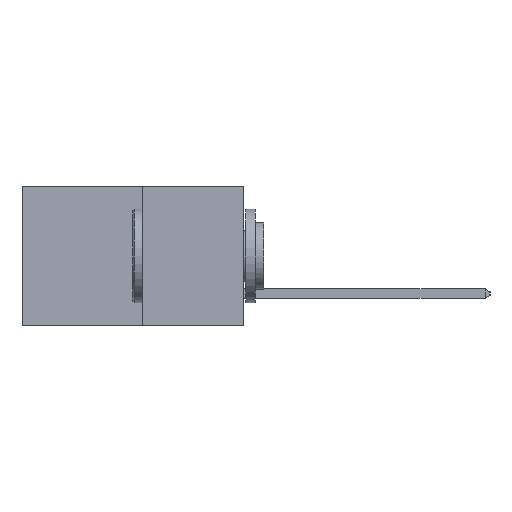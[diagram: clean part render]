
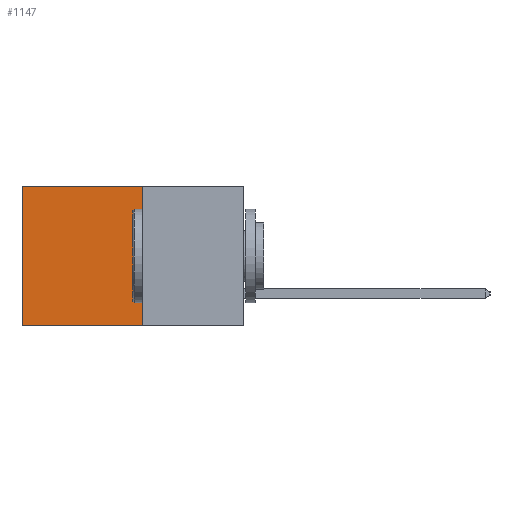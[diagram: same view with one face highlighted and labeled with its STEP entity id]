
A CAD part, left-side view. The second image highlights one B-rep face of the part: STEP entity #1147.
In plain terms, the highlighted planar face has unit normal (-1, 0, 0).
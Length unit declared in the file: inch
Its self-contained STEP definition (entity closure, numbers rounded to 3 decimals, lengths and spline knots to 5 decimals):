
#258 = EDGE_CURVE ( 'NONE', #2071, #15005, #1141, .T. ) ;
#296 = VECTOR ( 'NONE', #12312, 39.37008 ) ;
#369 = CARTESIAN_POINT ( 'NONE',  ( 0.277, 0.27, -0.37 ) ) ;
#683 = ORIENTED_EDGE ( 'NONE', *, *, #8868, .F. ) ;
#814 = LINE ( 'NONE', #369, #4011 ) ;
#1141 = LINE ( 'NONE', #3238, #7914 ) ;
#1147 = ADVANCED_FACE ( 'NONE', ( #5329 ), #16847, .F. ) ;
#1231 = EDGE_LOOP ( 'NONE', ( #7784, #683, #7365, #6443 ) ) ;
#1755 = CARTESIAN_POINT ( 'NONE',  ( 0.277, 0.27, -0.37 ) ) ;
#2071 = VERTEX_POINT ( 'NONE', #8346 ) ;
#2297 = CARTESIAN_POINT ( 'NONE',  ( 0.277, 0.59, 0. ) ) ;
#3066 = DIRECTION ( 'NONE',  ( 0., 1., 0. ) ) ;
#3147 = DIRECTION ( 'NONE',  ( 0., 0., -1. ) ) ;
#3178 = CARTESIAN_POINT ( 'NONE',  ( 0.277, 0.27, 0. ) ) ;
#3238 = CARTESIAN_POINT ( 'NONE',  ( 0.277, 0.27, -0.37 ) ) ;
#3943 = AXIS2_PLACEMENT_3D ( 'NONE', #1755, #9935, #10666 ) ;
#4011 = VECTOR ( 'NONE', #3066, 39.37008 ) ;
#4597 = VERTEX_POINT ( 'NONE', #2297 ) ;
#4773 = CARTESIAN_POINT ( 'NONE',  ( 0.277, 0.27, -0.37 ) ) ;
#5329 = FACE_OUTER_BOUND ( 'NONE', #1231, .T. ) ;
#6443 = ORIENTED_EDGE ( 'NONE', *, *, #8916, .T. ) ;
#7365 = ORIENTED_EDGE ( 'NONE', *, *, #258, .F. ) ;
#7784 = ORIENTED_EDGE ( 'NONE', *, *, #11044, .T. ) ;
#7914 = VECTOR ( 'NONE', #3147, 39.37008 ) ;
#8346 = CARTESIAN_POINT ( 'NONE',  ( 0.277, 0.27, 0. ) ) ;
#8868 = EDGE_CURVE ( 'NONE', #15005, #10416, #814, .T. ) ;
#8916 = EDGE_CURVE ( 'NONE', #2071, #4597, #10827, .T. ) ;
#9935 = DIRECTION ( 'NONE',  ( 1., 0., 0. ) ) ;
#9945 = DIRECTION ( 'NONE',  ( 0., 1., 0. ) ) ;
#10380 = VECTOR ( 'NONE', #9945, 39.37008 ) ;
#10416 = VERTEX_POINT ( 'NONE', #14678 ) ;
#10666 = DIRECTION ( 'NONE',  ( 0., 0., -1. ) ) ;
#10827 = LINE ( 'NONE', #3178, #10380 ) ;
#10931 = CARTESIAN_POINT ( 'NONE',  ( 0.277, 0.59, -0.37 ) ) ;
#11044 = EDGE_CURVE ( 'NONE', #4597, #10416, #11150, .T. ) ;
#11150 = LINE ( 'NONE', #10931, #296 ) ;
#12312 = DIRECTION ( 'NONE',  ( 0., 0., -1. ) ) ;
#14678 = CARTESIAN_POINT ( 'NONE',  ( 0.277, 0.59, -0.37 ) ) ;
#15005 = VERTEX_POINT ( 'NONE', #4773 ) ;
#16847 = PLANE ( 'NONE',  #3943 ) ;
